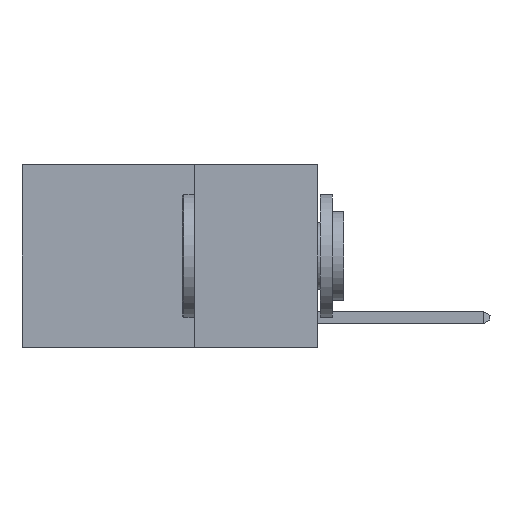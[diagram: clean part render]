
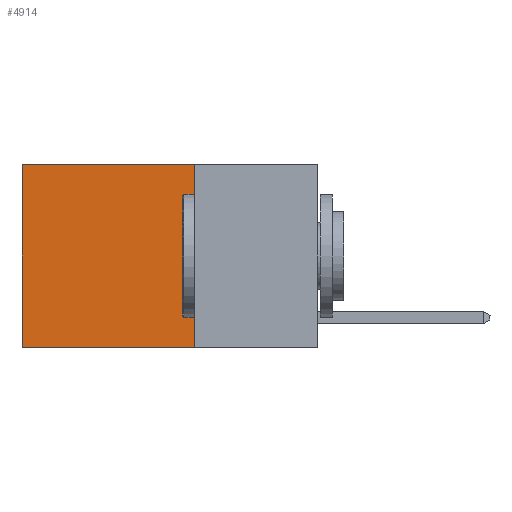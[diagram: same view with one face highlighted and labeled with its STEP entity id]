
A CAD part, left-side view. The second image highlights one B-rep face of the part: STEP entity #4914.
In plain terms, the highlighted planar face has unit normal (-1, 0, 0).
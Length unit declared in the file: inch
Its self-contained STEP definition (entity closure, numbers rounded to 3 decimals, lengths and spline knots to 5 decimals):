
#126 = VECTOR ( 'NONE', #9777, 39.37008 ) ;
#617 = FACE_OUTER_BOUND ( 'NONE', #6337, .T. ) ;
#818 = VECTOR ( 'NONE', #13083, 39.37008 ) ;
#879 = CARTESIAN_POINT ( 'NONE',  ( 0.2625, 0.25, -0.37 ) ) ;
#908 = VECTOR ( 'NONE', #917, 39.37008 ) ;
#917 = DIRECTION ( 'NONE',  ( 0., 1., 0. ) ) ;
#1639 = EDGE_CURVE ( 'NONE', #5384, #12955, #7879, .T. ) ;
#2135 = EDGE_CURVE ( 'NONE', #6914, #12955, #5619, .T. ) ;
#3931 = DIRECTION ( 'NONE',  ( 0., 0., -1. ) ) ;
#3958 = CARTESIAN_POINT ( 'NONE',  ( 0.2625, 0.25, 0. ) ) ;
#4570 = ORIENTED_EDGE ( 'NONE', *, *, #2135, .T. ) ;
#4914 = ADVANCED_FACE ( 'NONE', ( #617 ), #6084, .F. ) ;
#5384 = VERTEX_POINT ( 'NONE', #7222 ) ;
#5619 = LINE ( 'NONE', #7172, #10933 ) ;
#5890 = LINE ( 'NONE', #13185, #818 ) ;
#6084 = PLANE ( 'NONE',  #8498 ) ;
#6147 = VERTEX_POINT ( 'NONE', #12244 ) ;
#6337 = EDGE_LOOP ( 'NONE', ( #4570, #12825, #6500, #10247 ) ) ;
#6500 = ORIENTED_EDGE ( 'NONE', *, *, #10376, .F. ) ;
#6914 = VERTEX_POINT ( 'NONE', #9666 ) ;
#7172 = CARTESIAN_POINT ( 'NONE',  ( 0.2625, 0.6, 0. ) ) ;
#7200 = DIRECTION ( 'NONE',  ( 0., 0., -1. ) ) ;
#7222 = CARTESIAN_POINT ( 'NONE',  ( 0.2625, 0.25, -0.37 ) ) ;
#7544 = CARTESIAN_POINT ( 'NONE',  ( 0.2625, 0.25, 0. ) ) ;
#7879 = LINE ( 'NONE', #879, #908 ) ;
#8498 = AXIS2_PLACEMENT_3D ( 'NONE', #3958, #13726, #7200 ) ;
#9666 = CARTESIAN_POINT ( 'NONE',  ( 0.2625, 0.6, 0. ) ) ;
#9777 = DIRECTION ( 'NONE',  ( 0., 1., 0. ) ) ;
#9999 = LINE ( 'NONE', #7544, #126 ) ;
#10247 = ORIENTED_EDGE ( 'NONE', *, *, #13275, .T. ) ;
#10295 = CARTESIAN_POINT ( 'NONE',  ( 0.2625, 0.6, -0.37 ) ) ;
#10376 = EDGE_CURVE ( 'NONE', #6147, #5384, #5890, .T. ) ;
#10933 = VECTOR ( 'NONE', #3931, 39.37008 ) ;
#12244 = CARTESIAN_POINT ( 'NONE',  ( 0.2625, 0.25, 0. ) ) ;
#12825 = ORIENTED_EDGE ( 'NONE', *, *, #1639, .F. ) ;
#12955 = VERTEX_POINT ( 'NONE', #10295 ) ;
#13083 = DIRECTION ( 'NONE',  ( 0., 0., -1. ) ) ;
#13185 = CARTESIAN_POINT ( 'NONE',  ( 0.2625, 0.25, 0. ) ) ;
#13275 = EDGE_CURVE ( 'NONE', #6147, #6914, #9999, .T. ) ;
#13726 = DIRECTION ( 'NONE',  ( 1., 0., 0. ) ) ;
